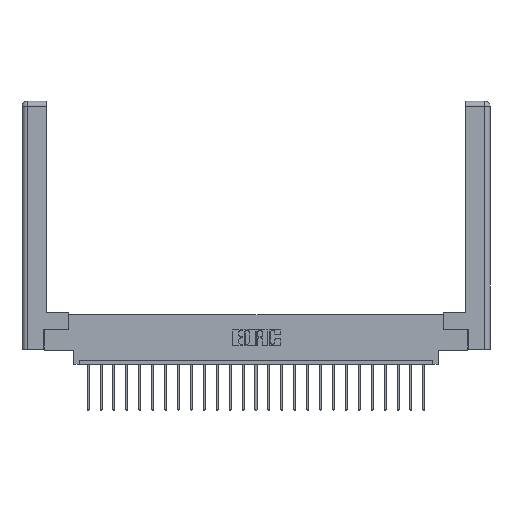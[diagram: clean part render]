
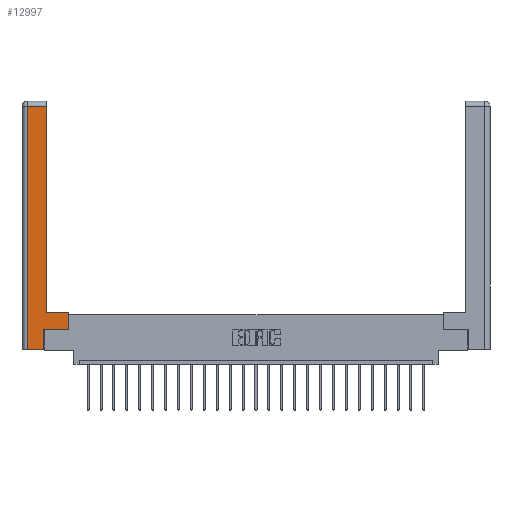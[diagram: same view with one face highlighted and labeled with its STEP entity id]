
A CAD part, top view. The second image highlights one B-rep face of the part: STEP entity #12997.
In plain terms, the highlighted planar face has unit normal (0, 0, 1).
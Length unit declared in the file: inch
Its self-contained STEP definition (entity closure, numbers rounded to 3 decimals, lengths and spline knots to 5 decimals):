
#101 = EDGE_LOOP ( 'NONE', ( #18707, #18434, #13760, #20607, #24664, #19199, #3794, #1803 ) ) ;
#192 = VECTOR ( 'NONE', #24703, 39.37008 ) ;
#633 = VERTEX_POINT ( 'NONE', #1842 ) ;
#1400 = VECTOR ( 'NONE', #3332, 39.37008 ) ;
#1695 = VECTOR ( 'NONE', #18203, 39.37008 ) ;
#1803 = ORIENTED_EDGE ( 'NONE', *, *, #8892, .T. ) ;
#1842 = CARTESIAN_POINT ( 'NONE',  ( 0.295, 2.94, 0. ) ) ;
#2932 = CARTESIAN_POINT ( 'NONE',  ( 0.265, 0.245, 0. ) ) ;
#3332 = DIRECTION ( 'NONE',  ( -1., 0., 0. ) ) ;
#3742 = CARTESIAN_POINT ( 'NONE',  ( 0.295, 3., 0. ) ) ;
#3794 = ORIENTED_EDGE ( 'NONE', *, *, #7966, .T. ) ;
#4529 = LINE ( 'NONE', #20309, #19174 ) ;
#4575 = CARTESIAN_POINT ( 'NONE',  ( 0.565, 0.45, 0. ) ) ;
#4703 = EDGE_CURVE ( 'NONE', #24592, #6174, #18217, .T. ) ;
#4888 = CARTESIAN_POINT ( 'NONE',  ( 0.265, 0., 0. ) ) ;
#5301 = EDGE_CURVE ( 'NONE', #6174, #5418, #11089, .T. ) ;
#5418 = VERTEX_POINT ( 'NONE', #12878 ) ;
#5927 = LINE ( 'NONE', #3742, #20822 ) ;
#6174 = VERTEX_POINT ( 'NONE', #13176 ) ;
#7218 = AXIS2_PLACEMENT_3D ( 'NONE', #10852, #14669, #23978 ) ;
#7460 = LINE ( 'NONE', #9255, #1400 ) ;
#7966 = EDGE_CURVE ( 'NONE', #5418, #23532, #15270, .T. ) ;
#8756 = VERTEX_POINT ( 'NONE', #10245 ) ;
#8892 = EDGE_CURVE ( 'NONE', #23532, #10642, #23539, .T. ) ;
#9189 = EDGE_CURVE ( 'NONE', #10642, #633, #5927, .T. ) ;
#9255 = CARTESIAN_POINT ( 'NONE',  ( 0.0615, 2.94, 0. ) ) ;
#9668 = EDGE_CURVE ( 'NONE', #17222, #24592, #4529, .T. ) ;
#10230 = VECTOR ( 'NONE', #10908, 39.37008 ) ;
#10245 = CARTESIAN_POINT ( 'NONE',  ( 0.0615, 2.94, 0. ) ) ;
#10642 = VERTEX_POINT ( 'NONE', #22164 ) ;
#10852 = CARTESIAN_POINT ( 'NONE',  ( 0., 0., 0. ) ) ;
#10908 = DIRECTION ( 'NONE',  ( 0., -1., 0. ) ) ;
#11089 = LINE ( 'NONE', #18942, #192 ) ;
#11994 = VECTOR ( 'NONE', #23796, 39.37008 ) ;
#12508 = PLANE ( 'NONE',  #7218 ) ;
#12748 = FACE_OUTER_BOUND ( 'NONE', #101, .T. ) ;
#12794 = DIRECTION ( 'NONE',  ( 1., 0., 0. ) ) ;
#12878 = CARTESIAN_POINT ( 'NONE',  ( 0.565, 0.245, 0. ) ) ;
#12997 = ADVANCED_FACE ( 'NONE', ( #12748 ), #12508, .F. ) ;
#13176 = CARTESIAN_POINT ( 'NONE',  ( 0.265, 0.245, 0. ) ) ;
#13545 = CARTESIAN_POINT ( 'NONE',  ( 0.0615, 0., 0. ) ) ;
#13760 = ORIENTED_EDGE ( 'NONE', *, *, #14507, .T. ) ;
#14507 = EDGE_CURVE ( 'NONE', #8756, #17222, #19713, .T. ) ;
#14669 = DIRECTION ( 'NONE',  ( 0., 0., -1. ) ) ;
#15270 = LINE ( 'NONE', #18043, #11994 ) ;
#17222 = VERTEX_POINT ( 'NONE', #13545 ) ;
#18043 = CARTESIAN_POINT ( 'NONE',  ( 0.565, 0.45, 0. ) ) ;
#18069 = DIRECTION ( 'NONE',  ( 0., 1., 0. ) ) ;
#18203 = DIRECTION ( 'NONE',  ( -1., 0., 0. ) ) ;
#18217 = LINE ( 'NONE', #2932, #19416 ) ;
#18434 = ORIENTED_EDGE ( 'NONE', *, *, #19783, .T. ) ;
#18707 = ORIENTED_EDGE ( 'NONE', *, *, #9189, .T. ) ;
#18942 = CARTESIAN_POINT ( 'NONE',  ( 0.565, 0.245, 0. ) ) ;
#19174 = VECTOR ( 'NONE', #12794, 39.37008 ) ;
#19199 = ORIENTED_EDGE ( 'NONE', *, *, #5301, .T. ) ;
#19416 = VECTOR ( 'NONE', #18069, 39.37008 ) ;
#19713 = LINE ( 'NONE', #22446, #10230 ) ;
#19783 = EDGE_CURVE ( 'NONE', #633, #8756, #7460, .T. ) ;
#19933 = CARTESIAN_POINT ( 'NONE',  ( 0.295, 0.45, 0. ) ) ;
#20309 = CARTESIAN_POINT ( 'NONE',  ( 0.265, 0., 0. ) ) ;
#20607 = ORIENTED_EDGE ( 'NONE', *, *, #9668, .T. ) ;
#20822 = VECTOR ( 'NONE', #24704, 39.37008 ) ;
#22164 = CARTESIAN_POINT ( 'NONE',  ( 0.295, 0.45, 0. ) ) ;
#22446 = CARTESIAN_POINT ( 'NONE',  ( 0.0615, 0., 0. ) ) ;
#23532 = VERTEX_POINT ( 'NONE', #4575 ) ;
#23539 = LINE ( 'NONE', #19933, #1695 ) ;
#23796 = DIRECTION ( 'NONE',  ( 0., 1., 0. ) ) ;
#23978 = DIRECTION ( 'NONE',  ( -1., 0., 0. ) ) ;
#24592 = VERTEX_POINT ( 'NONE', #4888 ) ;
#24664 = ORIENTED_EDGE ( 'NONE', *, *, #4703, .T. ) ;
#24703 = DIRECTION ( 'NONE',  ( 1., 0., 0. ) ) ;
#24704 = DIRECTION ( 'NONE',  ( 0., 1., 0. ) ) ;
